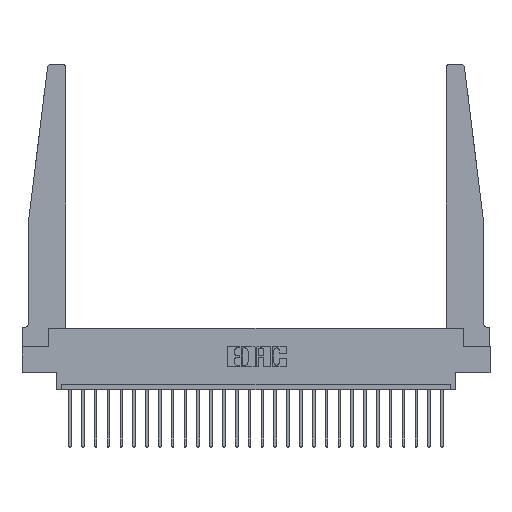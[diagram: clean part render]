
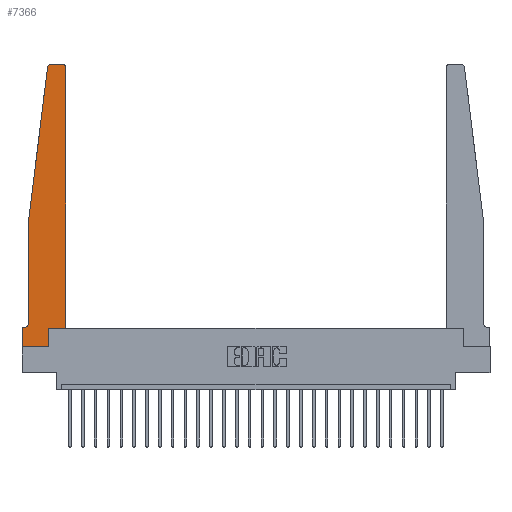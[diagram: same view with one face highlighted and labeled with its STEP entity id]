
A CAD part, top view. The second image highlights one B-rep face of the part: STEP entity #7366.
In plain terms, the highlighted planar face has unit normal (0, 0, 1).
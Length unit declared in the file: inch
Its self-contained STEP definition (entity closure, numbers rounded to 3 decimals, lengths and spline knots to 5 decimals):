
#5 = EDGE_CURVE ( 'NONE', #22962, #304, #14931, .T. ) ;
#233 = CIRCLE ( 'NONE', #19731, 0.05 ) ;
#304 = VERTEX_POINT ( 'NONE', #4943 ) ;
#837 = DIRECTION ( 'NONE',  ( 1., 0., 0. ) ) ;
#1119 = CARTESIAN_POINT ( 'NONE',  ( 0.425, 0.18, 0.37 ) ) ;
#1402 = EDGE_CURVE ( 'NONE', #1546, #23063, #23397, .T. ) ;
#1465 = ORIENTED_EDGE ( 'NONE', *, *, #9305, .T. ) ;
#1546 = VERTEX_POINT ( 'NONE', #10713 ) ;
#1777 = ORIENTED_EDGE ( 'NONE', *, *, #1402, .T. ) ;
#1933 = DIRECTION ( 'NONE',  ( -1., 0., 0. ) ) ;
#2078 = CARTESIAN_POINT ( 'NONE',  ( 0., 0.1875, 0.37 ) ) ;
#2123 = CARTESIAN_POINT ( 'NONE',  ( 0.425, 0.18, 0.37 ) ) ;
#2185 = VERTEX_POINT ( 'NONE', #22308 ) ;
#2527 = CARTESIAN_POINT ( 'NONE',  ( 0.065, 1.25, 0.37 ) ) ;
#2648 = CARTESIAN_POINT ( 'NONE',  ( 0.425, 0.18, 0.37 ) ) ;
#2699 = VECTOR ( 'NONE', #19494, 39.37008 ) ;
#3045 = CARTESIAN_POINT ( 'NONE',  ( 0.27653, 2.75, 0.37 ) ) ;
#3460 = EDGE_CURVE ( 'NONE', #304, #11536, #13578, .T. ) ;
#3929 = DIRECTION ( 'NONE',  ( 0., -1., 0. ) ) ;
#4147 = LINE ( 'NONE', #15557, #15688 ) ;
#4695 = AXIS2_PLACEMENT_3D ( 'NONE', #17168, #19323, #15110 ) ;
#4862 = EDGE_CURVE ( 'NONE', #10232, #8772, #7733, .T. ) ;
#4943 = CARTESIAN_POINT ( 'NONE',  ( 0., 0., 0.37 ) ) ;
#4962 = CARTESIAN_POINT ( 'NONE',  ( 0.2605, 0., 0.37 ) ) ;
#5014 = EDGE_CURVE ( 'NONE', #11536, #1546, #13504, .T. ) ;
#5178 = ORIENTED_EDGE ( 'NONE', *, *, #7606, .T. ) ;
#5755 = CARTESIAN_POINT ( 'NONE',  ( 0.24675, 2.72367, 0.37 ) ) ;
#5912 = VECTOR ( 'NONE', #8921, 39.37008 ) ;
#5929 = VERTEX_POINT ( 'NONE', #8153 ) ;
#6555 = FACE_OUTER_BOUND ( 'NONE', #9923, .T. ) ;
#6644 = EDGE_CURVE ( 'NONE', #11963, #12289, #11447, .T. ) ;
#6757 = CARTESIAN_POINT ( 'NONE',  ( 0., 0., 0.37 ) ) ;
#7366 = ADVANCED_FACE ( 'NONE', ( #6555 ), #13344, .T. ) ;
#7606 = EDGE_CURVE ( 'NONE', #12289, #20219, #21688, .T. ) ;
#7653 = EDGE_CURVE ( 'NONE', #23063, #10232, #23871, .T. ) ;
#7708 = LINE ( 'NONE', #10255, #17682 ) ;
#7733 = CIRCLE ( 'NONE', #13129, 0.03 ) ;
#8037 = LINE ( 'NONE', #10386, #22651 ) ;
#8153 = CARTESIAN_POINT ( 'NONE',  ( 0.065, 0.2375, 0.37 ) ) ;
#8506 = DIRECTION ( 'NONE',  ( -1., 0., 0. ) ) ;
#8544 = ORIENTED_EDGE ( 'NONE', *, *, #4862, .T. ) ;
#8772 = VERTEX_POINT ( 'NONE', #21779 ) ;
#8793 = ORIENTED_EDGE ( 'NONE', *, *, #20539, .T. ) ;
#8820 = CARTESIAN_POINT ( 'NONE',  ( 0.395, 2.72, 0.37 ) ) ;
#8921 = DIRECTION ( 'NONE',  ( 0., 1., 0. ) ) ;
#9305 = EDGE_CURVE ( 'NONE', #8772, #11963, #7708, .T. ) ;
#9681 = DIRECTION ( 'NONE',  ( 0., 0., -1. ) ) ;
#9737 = DIRECTION ( 'NONE',  ( 0., 1., 0. ) ) ;
#9923 = EDGE_LOOP ( 'NONE', ( #1465, #19369, #5178, #8793, #24804, #13945, #20736, #22609, #19458, #1777, #11062, #8544 ) ) ;
#10232 = VERTEX_POINT ( 'NONE', #15258 ) ;
#10255 = CARTESIAN_POINT ( 'NONE',  ( 0.25, 2.75, 0.37 ) ) ;
#10270 = CARTESIAN_POINT ( 'NONE',  ( 0.065, 1.25, 0.37 ) ) ;
#10386 = CARTESIAN_POINT ( 'NONE',  ( 0.065, 0.1875, 0.37 ) ) ;
#10713 = CARTESIAN_POINT ( 'NONE',  ( 0.2605, 0.18, 0.37 ) ) ;
#11062 = ORIENTED_EDGE ( 'NONE', *, *, #7653, .T. ) ;
#11447 = CIRCLE ( 'NONE', #21234, 0.03 ) ;
#11536 = VERTEX_POINT ( 'NONE', #4962 ) ;
#11856 = CARTESIAN_POINT ( 'NONE',  ( 0., 0., 0.37 ) ) ;
#11963 = VERTEX_POINT ( 'NONE', #3045 ) ;
#12289 = VERTEX_POINT ( 'NONE', #5755 ) ;
#13129 = AXIS2_PLACEMENT_3D ( 'NONE', #8820, #22382, #24360 ) ;
#13344 = PLANE ( 'NONE',  #4695 ) ;
#13504 = LINE ( 'NONE', #15478, #17726 ) ;
#13523 = VECTOR ( 'NONE', #19999, 39.37008 ) ;
#13578 = LINE ( 'NONE', #11856, #14769 ) ;
#13945 = ORIENTED_EDGE ( 'NONE', *, *, #22340, .T. ) ;
#14769 = VECTOR ( 'NONE', #15997, 39.37008 ) ;
#14931 = LINE ( 'NONE', #6757, #17650 ) ;
#15110 = DIRECTION ( 'NONE',  ( 1., 0., 0. ) ) ;
#15258 = CARTESIAN_POINT ( 'NONE',  ( 0.425, 2.72, 0.37 ) ) ;
#15478 = CARTESIAN_POINT ( 'NONE',  ( 0.2605, 0.18, 0.37 ) ) ;
#15557 = CARTESIAN_POINT ( 'NONE',  ( 0.065, 1.25, 0.37 ) ) ;
#15688 = VECTOR ( 'NONE', #3929, 39.37008 ) ;
#15997 = DIRECTION ( 'NONE',  ( 1., 0., 0. ) ) ;
#16005 = CARTESIAN_POINT ( 'NONE',  ( 0.27653, 2.72, 0.37 ) ) ;
#17168 = CARTESIAN_POINT ( 'NONE',  ( 0., 0.1875, 0.37 ) ) ;
#17650 = VECTOR ( 'NONE', #20121, 39.37008 ) ;
#17682 = VECTOR ( 'NONE', #17944, 39.37008 ) ;
#17726 = VECTOR ( 'NONE', #9737, 39.37008 ) ;
#17944 = DIRECTION ( 'NONE',  ( -1., 0., 0. ) ) ;
#19323 = DIRECTION ( 'NONE',  ( 0., 0., 1. ) ) ;
#19369 = ORIENTED_EDGE ( 'NONE', *, *, #6644, .T. ) ;
#19458 = ORIENTED_EDGE ( 'NONE', *, *, #5014, .T. ) ;
#19494 = DIRECTION ( 'NONE',  ( 1., 0., 0. ) ) ;
#19731 = AXIS2_PLACEMENT_3D ( 'NONE', #20759, #9681, #1933 ) ;
#19929 = EDGE_CURVE ( 'NONE', #5929, #2185, #233, .T. ) ;
#19999 = DIRECTION ( 'NONE',  ( -0.122, -0.992, 0. ) ) ;
#20121 = DIRECTION ( 'NONE',  ( 0., -1., 0. ) ) ;
#20219 = VERTEX_POINT ( 'NONE', #10270 ) ;
#20539 = EDGE_CURVE ( 'NONE', #20219, #5929, #4147, .T. ) ;
#20736 = ORIENTED_EDGE ( 'NONE', *, *, #5, .T. ) ;
#20759 = CARTESIAN_POINT ( 'NONE',  ( 0.015, 0.2375, 0.37 ) ) ;
#21234 = AXIS2_PLACEMENT_3D ( 'NONE', #16005, #22118, #837 ) ;
#21688 = LINE ( 'NONE', #2527, #13523 ) ;
#21779 = CARTESIAN_POINT ( 'NONE',  ( 0.395, 2.75, 0.37 ) ) ;
#22118 = DIRECTION ( 'NONE',  ( 0., 0., 1. ) ) ;
#22308 = CARTESIAN_POINT ( 'NONE',  ( 0.015, 0.1875, 0.37 ) ) ;
#22340 = EDGE_CURVE ( 'NONE', #2185, #22962, #8037, .T. ) ;
#22382 = DIRECTION ( 'NONE',  ( 0., 0., 1. ) ) ;
#22609 = ORIENTED_EDGE ( 'NONE', *, *, #3460, .T. ) ;
#22651 = VECTOR ( 'NONE', #8506, 39.37008 ) ;
#22962 = VERTEX_POINT ( 'NONE', #2078 ) ;
#23063 = VERTEX_POINT ( 'NONE', #2648 ) ;
#23397 = LINE ( 'NONE', #2123, #2699 ) ;
#23871 = LINE ( 'NONE', #1119, #5912 ) ;
#24360 = DIRECTION ( 'NONE',  ( 1., 0., 0. ) ) ;
#24804 = ORIENTED_EDGE ( 'NONE', *, *, #19929, .T. ) ;
